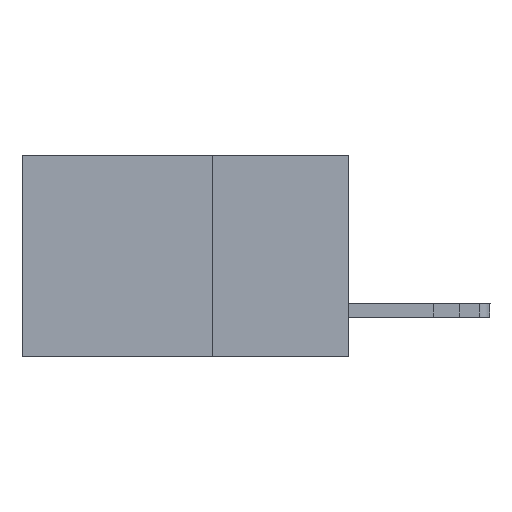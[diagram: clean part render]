
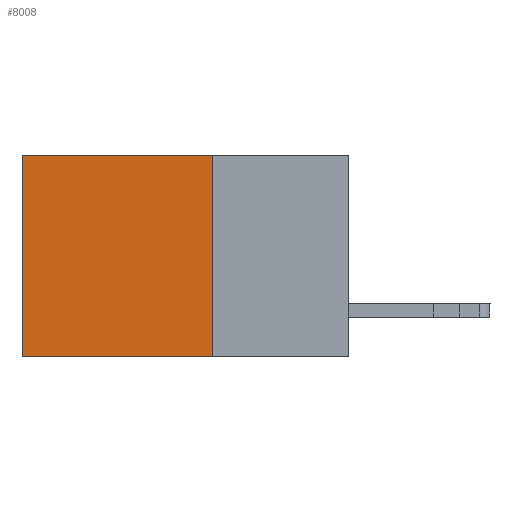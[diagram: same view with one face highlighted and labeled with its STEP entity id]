
A CAD part, left-side view. The second image highlights one B-rep face of the part: STEP entity #8008.
In plain terms, the highlighted planar face has unit normal (-1, 0, 0).
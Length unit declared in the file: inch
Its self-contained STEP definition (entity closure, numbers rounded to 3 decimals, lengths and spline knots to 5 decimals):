
#88 = VECTOR ( 'NONE', #3745, 39.37008 ) ;
#582 = DIRECTION ( 'NONE',  ( 0., 0., -1. ) ) ;
#697 = ORIENTED_EDGE ( 'NONE', *, *, #805, .T. ) ;
#805 = EDGE_CURVE ( 'NONE', #11998, #3491, #10136, .T. ) ;
#809 = ORIENTED_EDGE ( 'NONE', *, *, #8674, .F. ) ;
#965 = CARTESIAN_POINT ( 'NONE',  ( 0.298, 0.25, -0.37 ) ) ;
#2025 = CARTESIAN_POINT ( 'NONE',  ( 0.298, 0.25, -0.37 ) ) ;
#2474 = CARTESIAN_POINT ( 'NONE',  ( 0.298, 0.25, 0. ) ) ;
#2520 = VECTOR ( 'NONE', #5819, 39.37008 ) ;
#2630 = AXIS2_PLACEMENT_3D ( 'NONE', #2474, #10922, #582 ) ;
#3167 = CARTESIAN_POINT ( 'NONE',  ( 0.298, 0.6, -0.37 ) ) ;
#3253 = CARTESIAN_POINT ( 'NONE',  ( 0.298, 0.6, 0. ) ) ;
#3491 = VERTEX_POINT ( 'NONE', #3253 ) ;
#3683 = FACE_OUTER_BOUND ( 'NONE', #4631, .T. ) ;
#3745 = DIRECTION ( 'NONE',  ( 0., 1., 0. ) ) ;
#4487 = EDGE_CURVE ( 'NONE', #10372, #9082, #5219, .T. ) ;
#4539 = CARTESIAN_POINT ( 'NONE',  ( 0.298, 0.6, 0. ) ) ;
#4631 = EDGE_LOOP ( 'NONE', ( #5208, #10169, #809, #697 ) ) ;
#5208 = ORIENTED_EDGE ( 'NONE', *, *, #11056, .T. ) ;
#5219 = LINE ( 'NONE', #965, #88 ) ;
#5819 = DIRECTION ( 'NONE',  ( 0., 1., 0. ) ) ;
#8008 = ADVANCED_FACE ( 'NONE', ( #3683 ), #10810, .F. ) ;
#8621 = CARTESIAN_POINT ( 'NONE',  ( 0.298, 0.25, 0. ) ) ;
#8669 = LINE ( 'NONE', #4539, #10440 ) ;
#8674 = EDGE_CURVE ( 'NONE', #11998, #10372, #11729, .T. ) ;
#8914 = CARTESIAN_POINT ( 'NONE',  ( 0.298, 0.25, 0. ) ) ;
#9062 = CARTESIAN_POINT ( 'NONE',  ( 0.298, 0.25, 0. ) ) ;
#9082 = VERTEX_POINT ( 'NONE', #3167 ) ;
#10013 = DIRECTION ( 'NONE',  ( 0., 0., -1. ) ) ;
#10136 = LINE ( 'NONE', #8621, #2520 ) ;
#10169 = ORIENTED_EDGE ( 'NONE', *, *, #4487, .F. ) ;
#10251 = DIRECTION ( 'NONE',  ( 0., 0., -1. ) ) ;
#10372 = VERTEX_POINT ( 'NONE', #2025 ) ;
#10440 = VECTOR ( 'NONE', #10251, 39.37008 ) ;
#10702 = VECTOR ( 'NONE', #10013, 39.37008 ) ;
#10810 = PLANE ( 'NONE',  #2630 ) ;
#10922 = DIRECTION ( 'NONE',  ( 1., 0., 0. ) ) ;
#11056 = EDGE_CURVE ( 'NONE', #3491, #9082, #8669, .T. ) ;
#11729 = LINE ( 'NONE', #9062, #10702 ) ;
#11998 = VERTEX_POINT ( 'NONE', #8914 ) ;
